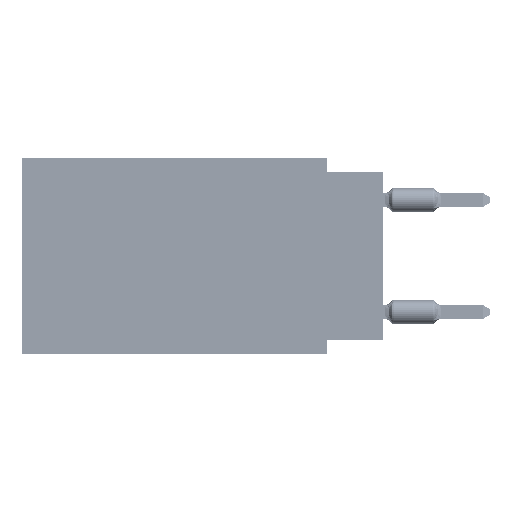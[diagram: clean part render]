
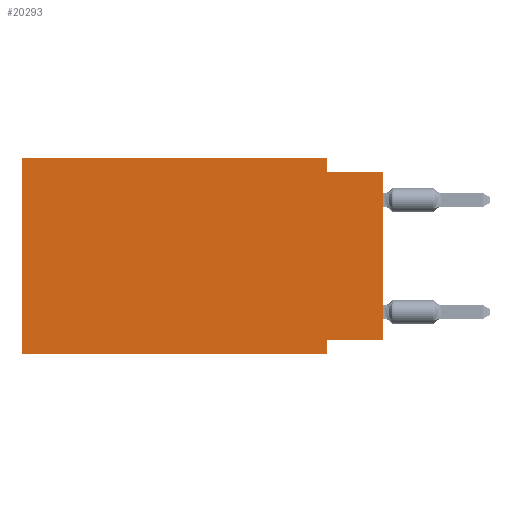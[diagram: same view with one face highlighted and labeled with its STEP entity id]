
A CAD part, left-side view. The second image highlights one B-rep face of the part: STEP entity #20293.
In plain terms, the highlighted planar face has unit normal (-1, 0, 0).
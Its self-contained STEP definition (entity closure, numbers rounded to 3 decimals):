
#1186 = VECTOR ( 'NONE', #85314, 1000. ) ;
#3982 = ORIENTED_EDGE ( 'NONE', *, *, #39492, .T. ) ;
#4268 = CARTESIAN_POINT ( 'NONE',  ( 0., 0., -0.635 ) ) ;
#5718 = FACE_OUTER_BOUND ( 'NONE', #7414, .T. ) ;
#5982 = CARTESIAN_POINT ( 'NONE',  ( 0., 2.54, 0. ) ) ;
#7414 = EDGE_LOOP ( 'NONE', ( #3982, #60969, #62770, #78348, #14724, #51208, #45078, #18405 ) ) ;
#10219 = DIRECTION ( 'NONE',  ( 0., -1., 0. ) ) ;
#12314 = DIRECTION ( 'NONE',  ( 0., 0., -1. ) ) ;
#13128 = DIRECTION ( 'NONE',  ( 0., -1., 0. ) ) ;
#14724 = ORIENTED_EDGE ( 'NONE', *, *, #32747, .F. ) ;
#18405 = ORIENTED_EDGE ( 'NONE', *, *, #67756, .F. ) ;
#20293 = ADVANCED_FACE ( 'NONE', ( #5718 ), #34221, .F. ) ;
#20784 = CARTESIAN_POINT ( 'NONE',  ( 0., 2.54, -0.635 ) ) ;
#20812 = CARTESIAN_POINT ( 'NONE',  ( 0., 2.54, 0. ) ) ;
#25153 = CARTESIAN_POINT ( 'NONE',  ( 0., 2.54, -8.255 ) ) ;
#27205 = DIRECTION ( 'NONE',  ( 1., 0., 0. ) ) ;
#30343 = CARTESIAN_POINT ( 'NONE',  ( 0., 0., -8.255 ) ) ;
#31966 = CARTESIAN_POINT ( 'NONE',  ( 0., 2.54, -8.89 ) ) ;
#32747 = EDGE_CURVE ( 'NONE', #40304, #53677, #76467, .T. ) ;
#34221 = PLANE ( 'NONE',  #85721 ) ;
#34600 = CARTESIAN_POINT ( 'NONE',  ( 0., 2.54, -8.89 ) ) ;
#34840 = DIRECTION ( 'NONE',  ( 0., -1., 0. ) ) ;
#36056 = CARTESIAN_POINT ( 'NONE',  ( 0., 0., 0. ) ) ;
#38319 = VERTEX_POINT ( 'NONE', #34600 ) ;
#39107 = VECTOR ( 'NONE', #79041, 1000. ) ;
#39492 = EDGE_CURVE ( 'NONE', #66026, #73154, #73885, .T. ) ;
#40304 = VERTEX_POINT ( 'NONE', #80096 ) ;
#41789 = VERTEX_POINT ( 'NONE', #20812 ) ;
#42306 = CARTESIAN_POINT ( 'NONE',  ( 0., 16.383, -8.89 ) ) ;
#42871 = LINE ( 'NONE', #5982, #75753 ) ;
#45078 = ORIENTED_EDGE ( 'NONE', *, *, #63136, .F. ) ;
#46031 = EDGE_CURVE ( 'NONE', #53677, #41789, #50450, .T. ) ;
#49364 = CARTESIAN_POINT ( 'NONE',  ( 0., 16.383, 0. ) ) ;
#49616 = CARTESIAN_POINT ( 'NONE',  ( 0., 16.383, 0. ) ) ;
#50450 = LINE ( 'NONE', #75616, #76409 ) ;
#51208 = ORIENTED_EDGE ( 'NONE', *, *, #62946, .T. ) ;
#51828 = DIRECTION ( 'NONE',  ( 0., 1., 0. ) ) ;
#53194 = VECTOR ( 'NONE', #51828, 1000. ) ;
#53677 = VERTEX_POINT ( 'NONE', #84607 ) ;
#54841 = LINE ( 'NONE', #31966, #82688 ) ;
#60510 = CARTESIAN_POINT ( 'NONE',  ( 0., 0., -0.635 ) ) ;
#60969 = ORIENTED_EDGE ( 'NONE', *, *, #83042, .F. ) ;
#61267 = LINE ( 'NONE', #4268, #89208 ) ;
#62770 = ORIENTED_EDGE ( 'NONE', *, *, #82388, .F. ) ;
#62946 = EDGE_CURVE ( 'NONE', #40304, #38319, #77814, .T. ) ;
#62985 = DIRECTION ( 'NONE',  ( 0., 0., -1. ) ) ;
#63136 = EDGE_CURVE ( 'NONE', #64280, #38319, #54841, .T. ) ;
#64280 = VERTEX_POINT ( 'NONE', #25153 ) ;
#64822 = VERTEX_POINT ( 'NONE', #20784 ) ;
#66026 = VERTEX_POINT ( 'NONE', #30343 ) ;
#67756 = EDGE_CURVE ( 'NONE', #66026, #64280, #78938, .T. ) ;
#73154 = VERTEX_POINT ( 'NONE', #60510 ) ;
#73885 = LINE ( 'NONE', #36056, #39107 ) ;
#75616 = CARTESIAN_POINT ( 'NONE',  ( 0., 16.383, 0. ) ) ;
#75753 = VECTOR ( 'NONE', #62985, 1000. ) ;
#76409 = VECTOR ( 'NONE', #10219, 1000. ) ;
#76467 = LINE ( 'NONE', #49364, #1186 ) ;
#77196 = DIRECTION ( 'NONE',  ( 0., 0., -1. ) ) ;
#77814 = LINE ( 'NONE', #42306, #78150 ) ;
#78150 = VECTOR ( 'NONE', #34840, 1000. ) ;
#78348 = ORIENTED_EDGE ( 'NONE', *, *, #46031, .F. ) ;
#78487 = CARTESIAN_POINT ( 'NONE',  ( 0., 0., -8.255 ) ) ;
#78938 = LINE ( 'NONE', #78487, #53194 ) ;
#79041 = DIRECTION ( 'NONE',  ( 0., 0., 1. ) ) ;
#80096 = CARTESIAN_POINT ( 'NONE',  ( 0., 16.383, -8.89 ) ) ;
#82388 = EDGE_CURVE ( 'NONE', #41789, #64822, #42871, .T. ) ;
#82688 = VECTOR ( 'NONE', #12314, 1000. ) ;
#83042 = EDGE_CURVE ( 'NONE', #64822, #73154, #61267, .T. ) ;
#84607 = CARTESIAN_POINT ( 'NONE',  ( 0., 16.383, 0. ) ) ;
#85314 = DIRECTION ( 'NONE',  ( 0., 0., 1. ) ) ;
#85721 = AXIS2_PLACEMENT_3D ( 'NONE', #49616, #27205, #77196 ) ;
#89208 = VECTOR ( 'NONE', #13128, 1000. ) ;
